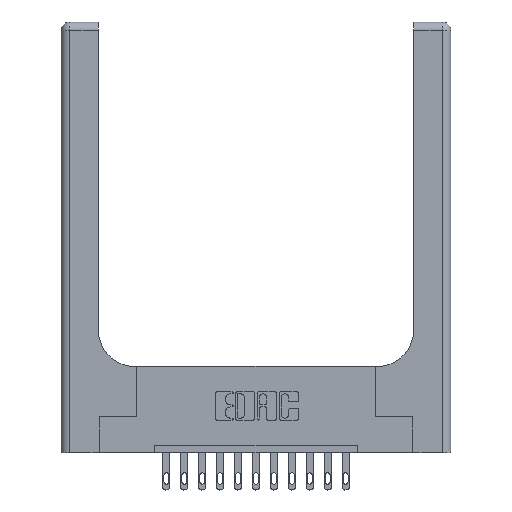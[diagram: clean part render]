
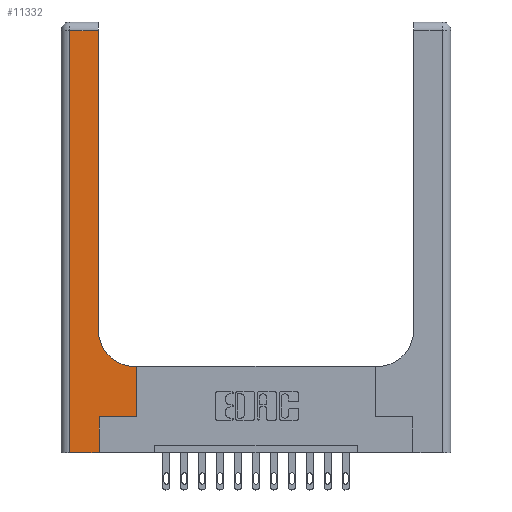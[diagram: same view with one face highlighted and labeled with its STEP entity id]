
A CAD part, top view. The second image highlights one B-rep face of the part: STEP entity #11332.
In plain terms, the highlighted planar face has unit normal (0, 0, 1).
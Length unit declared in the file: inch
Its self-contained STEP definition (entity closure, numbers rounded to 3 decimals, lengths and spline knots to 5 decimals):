
#261 = CARTESIAN_POINT ( 'NONE',  ( 0.26, 0.6, 0.37 ) ) ;
#485 = DIRECTION ( 'NONE',  ( -1., 0., 0. ) ) ;
#597 = LINE ( 'NONE', #9540, #4791 ) ;
#936 = EDGE_CURVE ( 'NONE', #15412, #1710, #7108, .T. ) ;
#1115 = VECTOR ( 'NONE', #12023, 39.37008 ) ;
#1149 = CARTESIAN_POINT ( 'NONE',  ( 0.06, 0., 0.37 ) ) ;
#1230 = DIRECTION ( 'NONE',  ( 0., -1., 0. ) ) ;
#1467 = VERTEX_POINT ( 'NONE', #3008 ) ;
#1710 = VERTEX_POINT ( 'NONE', #16117 ) ;
#1835 = VERTEX_POINT ( 'NONE', #7819 ) ;
#2017 = VERTEX_POINT ( 'NONE', #14825 ) ;
#2557 = CARTESIAN_POINT ( 'NONE',  ( 0.26, 0.85, 0.37 ) ) ;
#2817 = EDGE_CURVE ( 'NONE', #7723, #1467, #5730, .T. ) ;
#2876 = ORIENTED_EDGE ( 'NONE', *, *, #936, .T. ) ;
#3008 = CARTESIAN_POINT ( 'NONE',  ( 0.528, 0.6, 0.37 ) ) ;
#3297 = ORIENTED_EDGE ( 'NONE', *, *, #10282, .T. ) ;
#3361 = CARTESIAN_POINT ( 'NONE',  ( 0.265, 0., 0.37 ) ) ;
#3776 = EDGE_CURVE ( 'NONE', #1467, #4979, #12875, .T. ) ;
#4094 = CARTESIAN_POINT ( 'NONE',  ( 0.51, 0.6, 0.37 ) ) ;
#4199 = DIRECTION ( 'NONE',  ( 0., 0., -1. ) ) ;
#4260 = DIRECTION ( 'NONE',  ( 1., 0., 0. ) ) ;
#4405 = CARTESIAN_POINT ( 'NONE',  ( 0.528, 0.25, 0.37 ) ) ;
#4474 = LINE ( 'NONE', #8256, #10357 ) ;
#4687 = VERTEX_POINT ( 'NONE', #1149 ) ;
#4692 = CARTESIAN_POINT ( 'NONE',  ( 0.26, 3., 0.37 ) ) ;
#4791 = VECTOR ( 'NONE', #4260, 39.37008 ) ;
#4807 = LINE ( 'NONE', #8914, #12024 ) ;
#4979 = VERTEX_POINT ( 'NONE', #4094 ) ;
#5086 = LINE ( 'NONE', #11684, #6678 ) ;
#5188 = DIRECTION ( 'NONE',  ( -1., 0., 0. ) ) ;
#5343 = VECTOR ( 'NONE', #9730, 39.37008 ) ;
#5614 = DIRECTION ( 'NONE',  ( 0., 1., 0. ) ) ;
#5730 = LINE ( 'NONE', #4405, #1115 ) ;
#5769 = CARTESIAN_POINT ( 'NONE',  ( 0., 3., 0.37 ) ) ;
#6054 = EDGE_CURVE ( 'NONE', #1710, #2017, #4474, .T. ) ;
#6152 = CIRCLE ( 'NONE', #16331, 0.25 ) ;
#6678 = VECTOR ( 'NONE', #5614, 39.37008 ) ;
#6863 = DIRECTION ( 'NONE',  ( 1., 0., 0. ) ) ;
#7108 = LINE ( 'NONE', #4692, #8690 ) ;
#7288 = VECTOR ( 'NONE', #5188, 39.37008 ) ;
#7723 = VERTEX_POINT ( 'NONE', #8663 ) ;
#7819 = CARTESIAN_POINT ( 'NONE',  ( 0.265, 0.25, 0.37 ) ) ;
#8228 = FACE_OUTER_BOUND ( 'NONE', #16280, .T. ) ;
#8256 = CARTESIAN_POINT ( 'NONE',  ( 0., 2.94, 0.37 ) ) ;
#8403 = PLANE ( 'NONE',  #8577 ) ;
#8577 = AXIS2_PLACEMENT_3D ( 'NONE', #5769, #4199, #9476 ) ;
#8663 = CARTESIAN_POINT ( 'NONE',  ( 0.528, 0.25, 0.37 ) ) ;
#8690 = VECTOR ( 'NONE', #12145, 39.37008 ) ;
#8914 = CARTESIAN_POINT ( 'NONE',  ( 0.06, 3., 0.37 ) ) ;
#9061 = ORIENTED_EDGE ( 'NONE', *, *, #10490, .T. ) ;
#9476 = DIRECTION ( 'NONE',  ( -1., 0., 0. ) ) ;
#9540 = CARTESIAN_POINT ( 'NONE',  ( 0., 0., 0.37 ) ) ;
#9730 = DIRECTION ( 'NONE',  ( 1., 0., 0. ) ) ;
#10282 = EDGE_CURVE ( 'NONE', #1835, #7723, #12482, .T. ) ;
#10357 = VECTOR ( 'NONE', #485, 39.37008 ) ;
#10490 = EDGE_CURVE ( 'NONE', #4687, #15599, #597, .T. ) ;
#11332 = ADVANCED_FACE ( 'NONE', ( #8228 ), #8403, .F. ) ;
#11684 = CARTESIAN_POINT ( 'NONE',  ( 0.265, 0., 0.37 ) ) ;
#11760 = ORIENTED_EDGE ( 'NONE', *, *, #13070, .T. ) ;
#12023 = DIRECTION ( 'NONE',  ( 0., 1., 0. ) ) ;
#12024 = VECTOR ( 'NONE', #1230, 39.37008 ) ;
#12145 = DIRECTION ( 'NONE',  ( 0., 1., 0. ) ) ;
#12346 = ORIENTED_EDGE ( 'NONE', *, *, #6054, .T. ) ;
#12369 = ORIENTED_EDGE ( 'NONE', *, *, #2817, .T. ) ;
#12482 = LINE ( 'NONE', #14904, #5343 ) ;
#12777 = DIRECTION ( 'NONE',  ( 0., 0., -1. ) ) ;
#12875 = LINE ( 'NONE', #261, #7288 ) ;
#13070 = EDGE_CURVE ( 'NONE', #2017, #4687, #4807, .T. ) ;
#13582 = EDGE_CURVE ( 'NONE', #15599, #1835, #5086, .T. ) ;
#13630 = EDGE_CURVE ( 'NONE', #4979, #15412, #6152, .T. ) ;
#14825 = CARTESIAN_POINT ( 'NONE',  ( 0.06, 2.94, 0.37 ) ) ;
#14904 = CARTESIAN_POINT ( 'NONE',  ( 0.265, 0.25, 0.37 ) ) ;
#15368 = CARTESIAN_POINT ( 'NONE',  ( 0.51, 0.85, 0.37 ) ) ;
#15412 = VERTEX_POINT ( 'NONE', #2557 ) ;
#15472 = ORIENTED_EDGE ( 'NONE', *, *, #3776, .T. ) ;
#15599 = VERTEX_POINT ( 'NONE', #3361 ) ;
#15645 = ORIENTED_EDGE ( 'NONE', *, *, #13630, .T. ) ;
#15952 = ORIENTED_EDGE ( 'NONE', *, *, #13582, .T. ) ;
#16117 = CARTESIAN_POINT ( 'NONE',  ( 0.26, 2.94, 0.37 ) ) ;
#16280 = EDGE_LOOP ( 'NONE', ( #2876, #12346, #11760, #9061, #15952, #3297, #12369, #15472, #15645 ) ) ;
#16331 = AXIS2_PLACEMENT_3D ( 'NONE', #15368, #12777, #6863 ) ;
